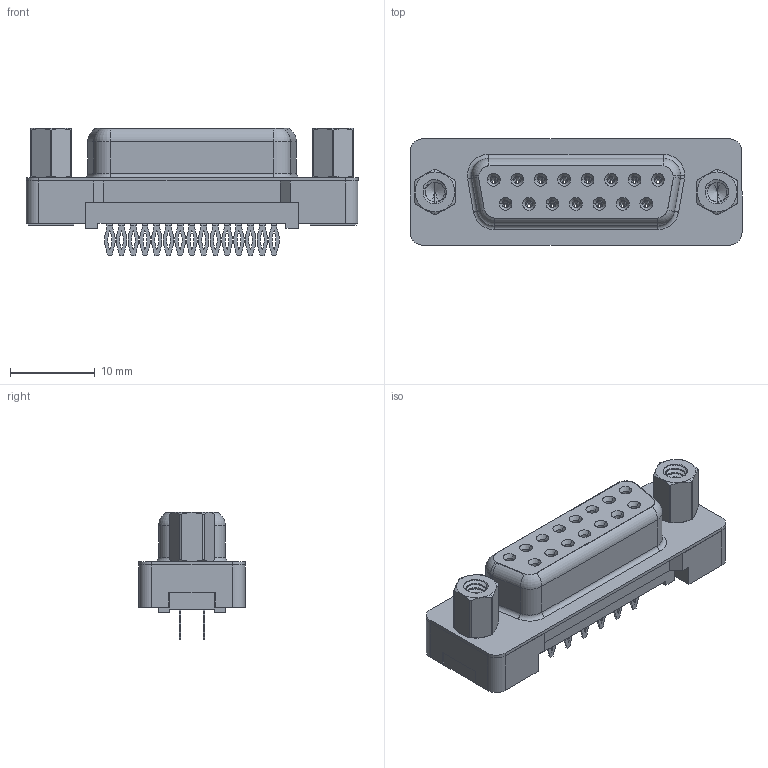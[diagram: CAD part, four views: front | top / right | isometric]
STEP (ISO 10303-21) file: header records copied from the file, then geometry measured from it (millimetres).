
FILE_DESCRIPTION (( 'STEP AP203' ), '1' );
FILE_NAME ('628-015-626-213.STEP', '2020-07-15T23:39:17', ( '' ), ( '' ), 'SwSTEP 2.0', 'SolidWorks 2020', '' );
FILE_SCHEMA (( 'CONFIG_CONTROL_DESIGN' ));
Length unit declared in the file: millimetre
Products named in the file (7): 628-015-626-213; 628 Plastic Body Housing_15 Contacts; 628 4-40 Hex Standoff; 628 PB 4-40 Threaded Rivet; 628 PB Contact Row 1_26; 628 PB Shell_15 Contacts; 628 PB Contact Row 2_26
Assembly tree (21 placements, depth 2):
  628-015-626-213
    628 Plastic Body Housing_15 Contacts
    628 PB Shell_15 Contacts
    628 PB Contact Row 1_26  x8
    628 PB Contact Row 2_26  x7
    628 PB 4-40 Threaded Rivet  x2
    628 4-40 Hex Standoff  x2
Bounding box: 39.2 x 12.55 x 15 mm (x, y, z)
Volume: 2663.5 mm3; surface area: 6386.4 mm2
Topology: 21 solids, 21 shells, 1721 faces, 4251 edges, 2598 vertices
Faces by surface type: plane 676, cylinder 476, bspline 348, torus 116, cone 105
Entity records: 23427 total; most frequent: CARTESIAN_POINT 9137, ORIENTED_EDGE 2834, DIRECTION 2591, EDGE_CURVE 1417, AXIS2_PLACEMENT_3D 901, VERTEX_POINT 888, VECTOR 789, LINE 789
